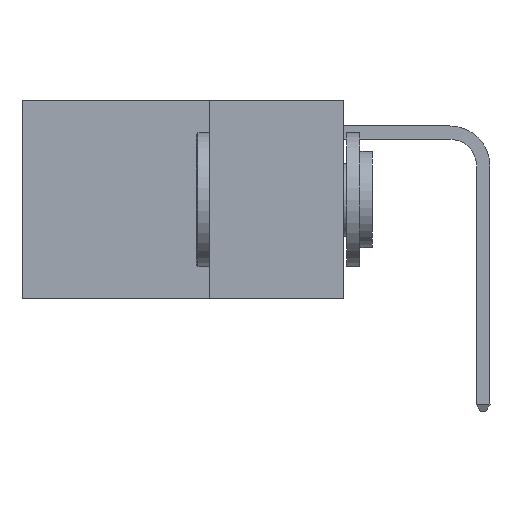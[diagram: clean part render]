
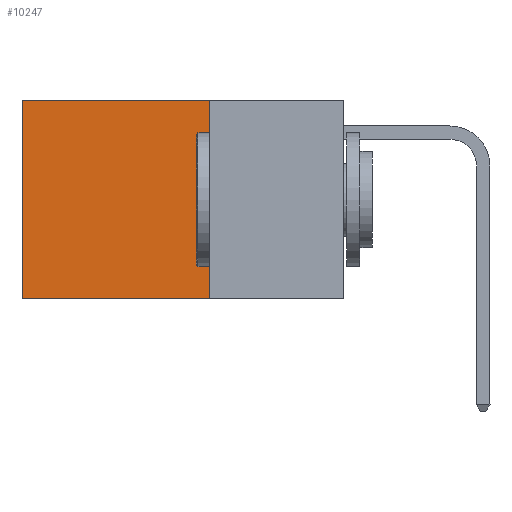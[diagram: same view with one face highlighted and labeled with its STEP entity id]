
A CAD part, left-side view. The second image highlights one B-rep face of the part: STEP entity #10247.
In plain terms, the highlighted planar face has unit normal (-1, 0, 0).
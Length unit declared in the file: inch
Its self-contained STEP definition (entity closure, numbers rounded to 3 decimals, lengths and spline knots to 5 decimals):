
#136 = DIRECTION ( 'NONE',  ( 0., 1., 0. ) ) ;
#161 = CARTESIAN_POINT ( 'NONE',  ( 0.2625, 0.25, -0.37 ) ) ;
#456 = DIRECTION ( 'NONE',  ( 0., 1., 0. ) ) ;
#655 = CARTESIAN_POINT ( 'NONE',  ( 0.2625, 0.25, 0. ) ) ;
#944 = DIRECTION ( 'NONE',  ( 0., 0., -1. ) ) ;
#965 = ORIENTED_EDGE ( 'NONE', *, *, #11276, .T. ) ;
#1038 = CARTESIAN_POINT ( 'NONE',  ( 0.2625, 0.6, 0. ) ) ;
#1305 = DIRECTION ( 'NONE',  ( 0., 0., -1. ) ) ;
#1406 = CARTESIAN_POINT ( 'NONE',  ( 0.2625, 0.6, -0.37 ) ) ;
#2252 = EDGE_LOOP ( 'NONE', ( #965, #5927, #10593, #7606 ) ) ;
#2358 = EDGE_CURVE ( 'NONE', #8513, #9508, #6112, .T. ) ;
#2612 = VERTEX_POINT ( 'NONE', #1406 ) ;
#4267 = AXIS2_PLACEMENT_3D ( 'NONE', #10192, #10178, #10175 ) ;
#4695 = CARTESIAN_POINT ( 'NONE',  ( 0.2625, 0.25, -0.37 ) ) ;
#5832 = EDGE_CURVE ( 'NONE', #8513, #9784, #7421, .T. ) ;
#5927 = ORIENTED_EDGE ( 'NONE', *, *, #11378, .F. ) ;
#6112 = LINE ( 'NONE', #655, #6198 ) ;
#6198 = VECTOR ( 'NONE', #456, 39.37008 ) ;
#7421 = LINE ( 'NONE', #11796, #7525 ) ;
#7525 = VECTOR ( 'NONE', #1305, 39.37008 ) ;
#7606 = ORIENTED_EDGE ( 'NONE', *, *, #2358, .T. ) ;
#8288 = CARTESIAN_POINT ( 'NONE',  ( 0.2625, 0.25, 0. ) ) ;
#8485 = VECTOR ( 'NONE', #136, 39.37008 ) ;
#8513 = VERTEX_POINT ( 'NONE', #8288 ) ;
#8547 = LINE ( 'NONE', #161, #8485 ) ;
#8754 = VECTOR ( 'NONE', #944, 39.37008 ) ;
#8769 = LINE ( 'NONE', #1038, #8754 ) ;
#9508 = VERTEX_POINT ( 'NONE', #10738 ) ;
#9784 = VERTEX_POINT ( 'NONE', #4695 ) ;
#10175 = DIRECTION ( 'NONE',  ( 0., 0., -1. ) ) ;
#10178 = DIRECTION ( 'NONE',  ( 1., 0., 0. ) ) ;
#10192 = CARTESIAN_POINT ( 'NONE',  ( 0.2625, 0.25, 0. ) ) ;
#10247 = ADVANCED_FACE ( 'NONE', ( #12457 ), #10288, .F. ) ;
#10288 = PLANE ( 'NONE',  #4267 ) ;
#10593 = ORIENTED_EDGE ( 'NONE', *, *, #5832, .F. ) ;
#10738 = CARTESIAN_POINT ( 'NONE',  ( 0.2625, 0.6, 0. ) ) ;
#11276 = EDGE_CURVE ( 'NONE', #9508, #2612, #8769, .T. ) ;
#11378 = EDGE_CURVE ( 'NONE', #9784, #2612, #8547, .T. ) ;
#11796 = CARTESIAN_POINT ( 'NONE',  ( 0.2625, 0.25, 0. ) ) ;
#12457 = FACE_OUTER_BOUND ( 'NONE', #2252, .T. ) ;
